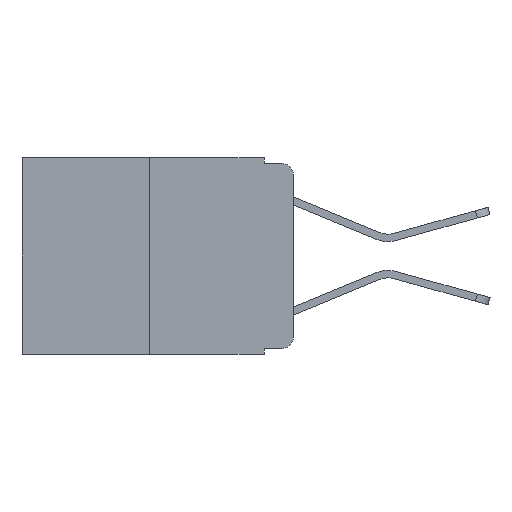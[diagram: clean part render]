
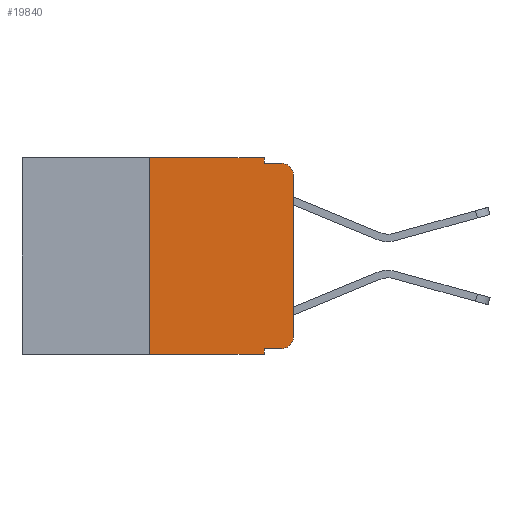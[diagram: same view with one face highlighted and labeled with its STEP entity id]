
A CAD part, left-side view. The second image highlights one B-rep face of the part: STEP entity #19840.
In plain terms, the highlighted planar face has unit normal (-1, 0, 0).
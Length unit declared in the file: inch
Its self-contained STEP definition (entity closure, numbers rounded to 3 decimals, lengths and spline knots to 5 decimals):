
#13 = VERTEX_POINT ( 'NONE', #11736 ) ;
#271 = FACE_OUTER_BOUND ( 'NONE', #18008, .T. ) ;
#955 = DIRECTION ( 'NONE',  ( 0., 0., -1. ) ) ;
#1094 = VERTEX_POINT ( 'NONE', #17667 ) ;
#1254 = VECTOR ( 'NONE', #13377, 39.37008 ) ;
#1312 = VECTOR ( 'NONE', #6606, 39.37008 ) ;
#1408 = CIRCLE ( 'NONE', #7526, 0.02 ) ;
#2023 = LINE ( 'NONE', #2554, #17208 ) ;
#2081 = LINE ( 'NONE', #14924, #16531 ) ;
#2188 = EDGE_CURVE ( 'NONE', #8278, #8700, #5926, .T. ) ;
#2200 = ORIENTED_EDGE ( 'NONE', *, *, #2456, .F. ) ;
#2456 = EDGE_CURVE ( 'NONE', #13, #1094, #19849, .T. ) ;
#2538 = CARTESIAN_POINT ( 'NONE',  ( 0., 0.473, 0. ) ) ;
#2554 = CARTESIAN_POINT ( 'NONE',  ( 0., 0.051, 0. ) ) ;
#2607 = DIRECTION ( 'NONE',  ( 0., 0., -1. ) ) ;
#2662 = CARTESIAN_POINT ( 'NONE',  ( 0., 0.051, -0.01 ) ) ;
#2746 = CARTESIAN_POINT ( 'NONE',  ( 0., 0.473, 0. ) ) ;
#3703 = EDGE_CURVE ( 'NONE', #5551, #19161, #9926, .T. ) ;
#3758 = EDGE_CURVE ( 'NONE', #14194, #8278, #2023, .T. ) ;
#3912 = CARTESIAN_POINT ( 'NONE',  ( 0., 0.02, -0.333 ) ) ;
#3934 = CARTESIAN_POINT ( 'NONE',  ( 0., 0., -0.313 ) ) ;
#4187 = CARTESIAN_POINT ( 'NONE',  ( 0., 0., -0.03 ) ) ;
#4234 = PLANE ( 'NONE',  #19871 ) ;
#4236 = DIRECTION ( 'NONE',  ( 0., -1., 0. ) ) ;
#4899 = AXIS2_PLACEMENT_3D ( 'NONE', #5812, #13641, #955 ) ;
#5507 = EDGE_CURVE ( 'NONE', #19161, #8700, #1408, .T. ) ;
#5551 = VERTEX_POINT ( 'NONE', #3934 ) ;
#5643 = CARTESIAN_POINT ( 'NONE',  ( 0., 0.25, 0. ) ) ;
#5761 = CARTESIAN_POINT ( 'NONE',  ( 0., 0.051, 0. ) ) ;
#5812 = CARTESIAN_POINT ( 'NONE',  ( 0., 0.02, -0.313 ) ) ;
#5926 = LINE ( 'NONE', #14928, #1312 ) ;
#5987 = DIRECTION ( 'NONE',  ( 0., 0., -1. ) ) ;
#6175 = VERTEX_POINT ( 'NONE', #12084 ) ;
#6312 = LINE ( 'NONE', #11489, #8868 ) ;
#6606 = DIRECTION ( 'NONE',  ( 0., -1., 0. ) ) ;
#6937 = DIRECTION ( 'NONE',  ( 0., -1., 0. ) ) ;
#7526 = AXIS2_PLACEMENT_3D ( 'NONE', #10370, #16891, #16820 ) ;
#7918 = LINE ( 'NONE', #14758, #1254 ) ;
#8278 = VERTEX_POINT ( 'NONE', #2662 ) ;
#8428 = DIRECTION ( 'NONE',  ( 0., 0., -1. ) ) ;
#8496 = CARTESIAN_POINT ( 'NONE',  ( 0., 0.051, 0. ) ) ;
#8700 = VERTEX_POINT ( 'NONE', #16239 ) ;
#8776 = EDGE_CURVE ( 'NONE', #6175, #1094, #6312, .T. ) ;
#8868 = VECTOR ( 'NONE', #17808, 39.37008 ) ;
#8874 = ORIENTED_EDGE ( 'NONE', *, *, #3703, .T. ) ;
#9210 = VECTOR ( 'NONE', #4236, 39.37008 ) ;
#9677 = VECTOR ( 'NONE', #18660, 39.37008 ) ;
#9926 = LINE ( 'NONE', #13739, #9677 ) ;
#10233 = VERTEX_POINT ( 'NONE', #5643 ) ;
#10370 = CARTESIAN_POINT ( 'NONE',  ( 0., 0.02, -0.03 ) ) ;
#10394 = ORIENTED_EDGE ( 'NONE', *, *, #12301, .F. ) ;
#11489 = CARTESIAN_POINT ( 'NONE',  ( 0., 0.473, -0.343 ) ) ;
#11736 = CARTESIAN_POINT ( 'NONE',  ( 0., 0.051, -0.333 ) ) ;
#11831 = ORIENTED_EDGE ( 'NONE', *, *, #13918, .F. ) ;
#12084 = CARTESIAN_POINT ( 'NONE',  ( 0., 0.25, -0.343 ) ) ;
#12301 = EDGE_CURVE ( 'NONE', #10233, #14194, #14754, .T. ) ;
#12745 = EDGE_CURVE ( 'NONE', #13391, #5551, #19822, .T. ) ;
#13030 = ORIENTED_EDGE ( 'NONE', *, *, #19147, .T. ) ;
#13377 = DIRECTION ( 'NONE',  ( 0., 0., 1. ) ) ;
#13391 = VERTEX_POINT ( 'NONE', #3912 ) ;
#13641 = DIRECTION ( 'NONE',  ( -1., 0., 0. ) ) ;
#13739 = CARTESIAN_POINT ( 'NONE',  ( 0., 0., 0. ) ) ;
#13918 = EDGE_CURVE ( 'NONE', #6175, #10233, #7918, .T. ) ;
#14194 = VERTEX_POINT ( 'NONE', #5761 ) ;
#14754 = LINE ( 'NONE', #2746, #9210 ) ;
#14758 = CARTESIAN_POINT ( 'NONE',  ( 0., 0.25, 0. ) ) ;
#14924 = CARTESIAN_POINT ( 'NONE',  ( 0., 0.051, -0.333 ) ) ;
#14928 = CARTESIAN_POINT ( 'NONE',  ( 0., 0.051, -0.01 ) ) ;
#15124 = ORIENTED_EDGE ( 'NONE', *, *, #5507, .T. ) ;
#15610 = ORIENTED_EDGE ( 'NONE', *, *, #12745, .T. ) ;
#16239 = CARTESIAN_POINT ( 'NONE',  ( 0., 0.02, -0.01 ) ) ;
#16531 = VECTOR ( 'NONE', #6937, 39.37008 ) ;
#16820 = DIRECTION ( 'NONE',  ( 0., 0., -1. ) ) ;
#16891 = DIRECTION ( 'NONE',  ( -1., 0., 0. ) ) ;
#17208 = VECTOR ( 'NONE', #5987, 39.37008 ) ;
#17667 = CARTESIAN_POINT ( 'NONE',  ( 0., 0.051, -0.343 ) ) ;
#17808 = DIRECTION ( 'NONE',  ( 0., -1., 0. ) ) ;
#18008 = EDGE_LOOP ( 'NONE', ( #8874, #15124, #18436, #18050, #10394, #11831, #18184, #2200, #13030, #15610 ) ) ;
#18050 = ORIENTED_EDGE ( 'NONE', *, *, #3758, .F. ) ;
#18184 = ORIENTED_EDGE ( 'NONE', *, *, #8776, .T. ) ;
#18436 = ORIENTED_EDGE ( 'NONE', *, *, #2188, .F. ) ;
#18660 = DIRECTION ( 'NONE',  ( 0., 0., 1. ) ) ;
#18712 = DIRECTION ( 'NONE',  ( 1., 0., 0. ) ) ;
#19147 = EDGE_CURVE ( 'NONE', #13, #13391, #2081, .T. ) ;
#19161 = VERTEX_POINT ( 'NONE', #4187 ) ;
#19337 = VECTOR ( 'NONE', #8428, 39.37008 ) ;
#19822 = CIRCLE ( 'NONE', #4899, 0.02 ) ;
#19840 = ADVANCED_FACE ( 'NONE', ( #271 ), #4234, .F. ) ;
#19849 = LINE ( 'NONE', #8496, #19337 ) ;
#19871 = AXIS2_PLACEMENT_3D ( 'NONE', #2538, #18712, #2607 ) ;
